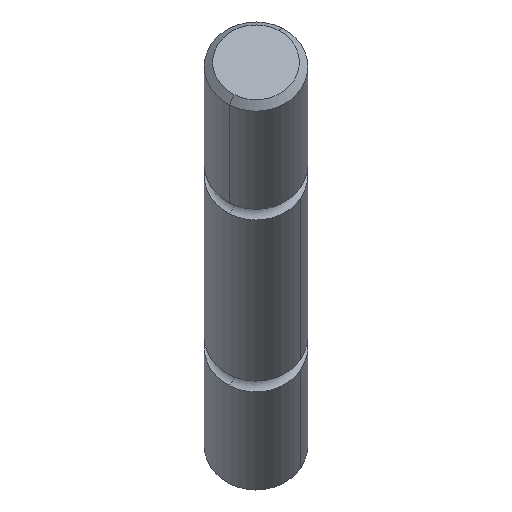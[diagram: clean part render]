
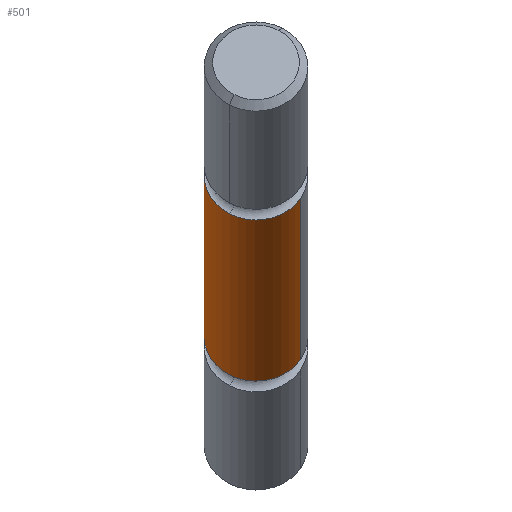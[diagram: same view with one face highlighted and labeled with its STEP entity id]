
A CAD part, front view. The second image highlights one B-rep face of the part: STEP entity #501.
In plain terms, the highlighted cylindrical face has radius 1.562 mm (diameter 3.124 mm), a partial arc.
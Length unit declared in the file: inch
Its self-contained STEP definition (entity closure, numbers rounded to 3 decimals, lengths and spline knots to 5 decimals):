
#37=CARTESIAN_POINT('',(3.4184,0.92687,-0.54889));
#38=DIRECTION('',(0.,-0.86,0.51));
#39=DIRECTION('',(-0.86,0.26,0.438));
#40=AXIS2_PLACEMENT_3D('',#37,#38,#39);
#53=DIRECTION('',(0.,-0.86,0.51));
#54=VECTOR('',#53,0.375);
#55=CARTESIAN_POINT('',(3.36549,1.2655,-0.713));
#56=LINE('',#55,#54);
#60=DIRECTION('',(0.,-0.86,0.51));
#61=VECTOR('',#60,0.375);
#62=CARTESIAN_POINT('',(3.47132,1.23356,-0.76693));
#63=LINE('',#62,#61);
#83=CARTESIAN_POINT('',(3.4184,1.24953,-0.73997));
#84=DIRECTION('',(0.,0.86,-0.51));
#85=DIRECTION('',(-0.51,-0.438,-0.74));
#86=AXIS2_PLACEMENT_3D('',#83,#84,#85);
#231=CARTESIAN_POINT('',(3.4184,1.24953,-0.73997));
#232=DIRECTION('',(0.,0.86,-0.51));
#233=DIRECTION('',(0.86,-0.26,-0.438));
#234=AXIS2_PLACEMENT_3D('',#231,#232,#233);
#279=CARTESIAN_POINT('',(3.4184,0.92687,
-0.54889));
#280=DIRECTION('',(0.,-0.86,0.51));
#281=DIRECTION('',(-0.51,-0.438,-0.74));
#282=AXIS2_PLACEMENT_3D('',#279,#280,#281);
#388=CARTESIAN_POINT('',(3.38707,0.8999,
-0.59442));
#390=VERTEX_POINT('',#388);
#397=CARTESIAN_POINT('',(3.38707,1.22257,-0.7855));
#398=VERTEX_POINT('',#397);
#407=CARTESIAN_POINT('',(3.47132,1.23356,-0.76693));
#408=CARTESIAN_POINT('',(3.47132,0.9109,
-0.57585));
#409=VERTEX_POINT('',#407);
#410=VERTEX_POINT('',#408);
#411=CARTESIAN_POINT('',(3.36549,1.2655,-0.713));
#412=CARTESIAN_POINT('',(3.36549,0.94284,
-0.52192));
#413=VERTEX_POINT('',#411);
#414=VERTEX_POINT('',#412);
#483=CARTESIAN_POINT('',(3.4184,1.24953,-0.73997));
#484=DIRECTION('',(0.,-0.86,0.51));
#485=DIRECTION('',(0.86,-0.26,-0.438));
#486=AXIS2_PLACEMENT_3D('',#483,#484,#485);
#487=CYLINDRICAL_SURFACE('',#486,0.0615);
#489=ORIENTED_EDGE('',*,*,#488,.T.);
#491=ORIENTED_EDGE('',*,*,#490,.T.);
#492=ORIENTED_EDGE('',*,*,#471,.T.);
#494=ORIENTED_EDGE('',*,*,#493,.T.);
#496=ORIENTED_EDGE('',*,*,#495,.F.);
#498=ORIENTED_EDGE('',*,*,#497,.T.);
#499=EDGE_LOOP('',(#489,#491,#492,#494,#496,#498));
#500=FACE_OUTER_BOUND('',#499,.F.);
#41=CIRCLE('',#40,0.0615);
#87=CIRCLE('',#86,0.0615);
#235=CIRCLE('',#234,0.0615);
#283=CIRCLE('',#282,0.0615);
#471=EDGE_CURVE('',#414,#390,#41,.T.);
#488=EDGE_CURVE('',#398,#413,#87,.T.);
#490=EDGE_CURVE('',#413,#414,#56,.T.);
#493=EDGE_CURVE('',#390,#410,#283,.T.);
#495=EDGE_CURVE('',#409,#410,#63,.T.);
#497=EDGE_CURVE('',#409,#398,#235,.T.);
#501=ADVANCED_FACE('',(#500),#487,.T.);
